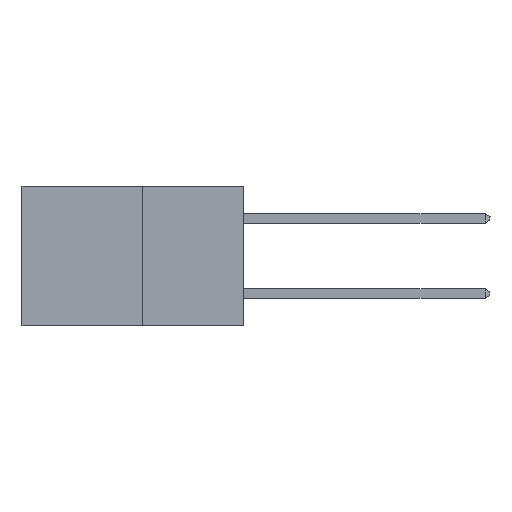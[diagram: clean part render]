
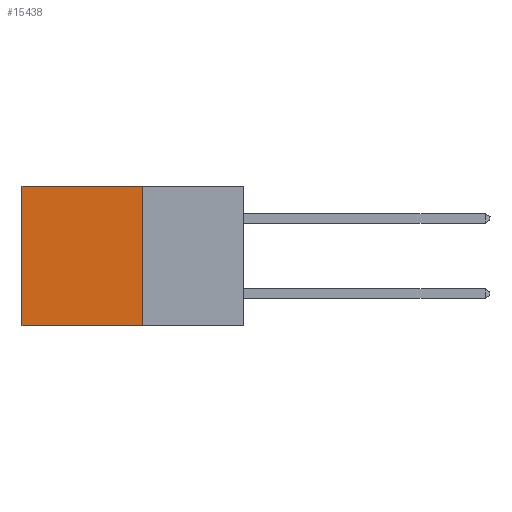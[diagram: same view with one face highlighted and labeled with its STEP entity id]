
A CAD part, left-side view. The second image highlights one B-rep face of the part: STEP entity #15438.
In plain terms, the highlighted planar face has unit normal (-1, 0, 0).
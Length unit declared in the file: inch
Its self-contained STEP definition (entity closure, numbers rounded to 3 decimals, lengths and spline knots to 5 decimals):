
#1814 = ORIENTED_EDGE ( 'NONE', *, *, #19160, .T. ) ;
#3627 = CARTESIAN_POINT ( 'NONE',  ( 0.277, 0.59, 0. ) ) ;
#4136 = CARTESIAN_POINT ( 'NONE',  ( 0.277, 0.27, -0.37 ) ) ;
#4162 = DIRECTION ( 'NONE',  ( 0., 0., -1. ) ) ;
#5180 = VERTEX_POINT ( 'NONE', #33561 ) ;
#8053 = CARTESIAN_POINT ( 'NONE',  ( 0.277, 0.27, -0.37 ) ) ;
#9383 = CARTESIAN_POINT ( 'NONE',  ( 0.277, 0.59, -0.37 ) ) ;
#9577 = CARTESIAN_POINT ( 'NONE',  ( 0.277, 0.27, -0.37 ) ) ;
#9591 = LINE ( 'NONE', #15584, #22719 ) ;
#9691 = EDGE_CURVE ( 'NONE', #29553, #5180, #30541, .T. ) ;
#11072 = VERTEX_POINT ( 'NONE', #3627 ) ;
#11983 = DIRECTION ( 'NONE',  ( 1., 0., 0. ) ) ;
#12201 = DIRECTION ( 'NONE',  ( 0., 1., 0. ) ) ;
#12960 = DIRECTION ( 'NONE',  ( 0., 1., 0. ) ) ;
#13528 = ORIENTED_EDGE ( 'NONE', *, *, #17612, .F. ) ;
#15438 = ADVANCED_FACE ( 'NONE', ( #20665 ), #27641, .F. ) ;
#15584 = CARTESIAN_POINT ( 'NONE',  ( 0.277, 0.27, 0. ) ) ;
#15818 = AXIS2_PLACEMENT_3D ( 'NONE', #4136, #11983, #30281 ) ;
#16246 = LINE ( 'NONE', #27667, #22410 ) ;
#16430 = VECTOR ( 'NONE', #4162, 39.37008 ) ;
#16633 = VECTOR ( 'NONE', #12201, 39.37008 ) ;
#17268 = LINE ( 'NONE', #9383, #16430 ) ;
#17612 = EDGE_CURVE ( 'NONE', #19448, #29553, #16246, .T. ) ;
#17623 = EDGE_LOOP ( 'NONE', ( #31302, #26916, #13528, #1814 ) ) ;
#19160 = EDGE_CURVE ( 'NONE', #19448, #11072, #9591, .T. ) ;
#19448 = VERTEX_POINT ( 'NONE', #21883 ) ;
#20665 = FACE_OUTER_BOUND ( 'NONE', #17623, .T. ) ;
#21883 = CARTESIAN_POINT ( 'NONE',  ( 0.277, 0.27, 0. ) ) ;
#22410 = VECTOR ( 'NONE', #22450, 39.37008 ) ;
#22450 = DIRECTION ( 'NONE',  ( 0., 0., -1. ) ) ;
#22719 = VECTOR ( 'NONE', #12960, 39.37008 ) ;
#26916 = ORIENTED_EDGE ( 'NONE', *, *, #9691, .F. ) ;
#27641 = PLANE ( 'NONE',  #15818 ) ;
#27667 = CARTESIAN_POINT ( 'NONE',  ( 0.277, 0.27, -0.37 ) ) ;
#29553 = VERTEX_POINT ( 'NONE', #8053 ) ;
#30281 = DIRECTION ( 'NONE',  ( 0., 0., -1. ) ) ;
#30541 = LINE ( 'NONE', #9577, #16633 ) ;
#31302 = ORIENTED_EDGE ( 'NONE', *, *, #33616, .T. ) ;
#33561 = CARTESIAN_POINT ( 'NONE',  ( 0.277, 0.59, -0.37 ) ) ;
#33616 = EDGE_CURVE ( 'NONE', #11072, #5180, #17268, .T. ) ;
